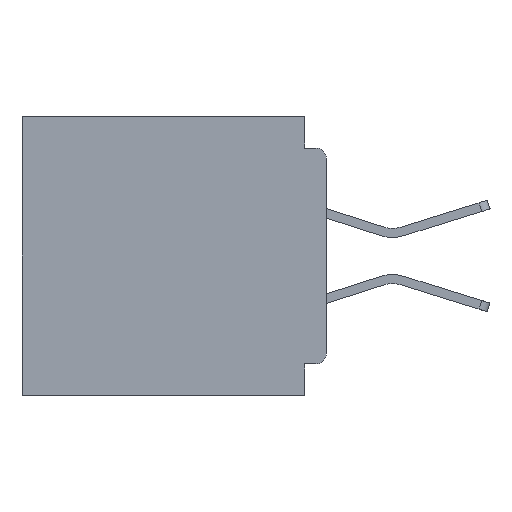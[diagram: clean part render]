
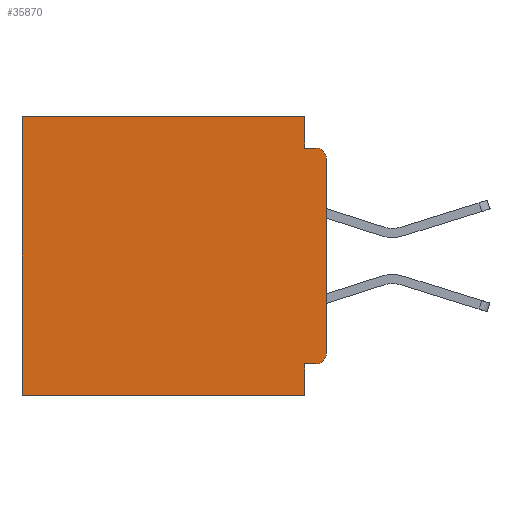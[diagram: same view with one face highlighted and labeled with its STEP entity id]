
A CAD part, left-side view. The second image highlights one B-rep face of the part: STEP entity #35870.
In plain terms, the highlighted planar face has unit normal (-1, 0, 0).
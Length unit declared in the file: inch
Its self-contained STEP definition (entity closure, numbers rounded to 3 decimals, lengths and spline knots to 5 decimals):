
#94 = VECTOR ( 'NONE', #45128, 39.37008 ) ;
#1416 = EDGE_LOOP ( 'NONE', ( #1685, #44539, #15303, #8636, #15761, #9876, #17056, #30043, #35942, #30133 ) ) ;
#1685 = ORIENTED_EDGE ( 'NONE', *, *, #7326, .F. ) ;
#1917 = VECTOR ( 'NONE', #26024, 39.37008 ) ;
#3438 = CARTESIAN_POINT ( 'NONE',  ( 0.3, 0.031, 0. ) ) ;
#3607 = PLANE ( 'NONE',  #48249 ) ;
#3907 = CARTESIAN_POINT ( 'NONE',  ( 0.3, 0.015, -0.355 ) ) ;
#5594 = CARTESIAN_POINT ( 'NONE',  ( 0.3, 0.015, -0.34 ) ) ;
#5842 = EDGE_CURVE ( 'NONE', #13653, #39688, #12678, .T. ) ;
#6872 = VECTOR ( 'NONE', #38490, 39.37008 ) ;
#7013 = VECTOR ( 'NONE', #7483, 39.37008 ) ;
#7326 = EDGE_CURVE ( 'NONE', #25076, #31655, #46342, .T. ) ;
#7483 = DIRECTION ( 'NONE',  ( 0., 0., -1. ) ) ;
#8036 = CARTESIAN_POINT ( 'NONE',  ( 0.3, 0.015, -0.06 ) ) ;
#8179 = VERTEX_POINT ( 'NONE', #11598 ) ;
#8214 = DIRECTION ( 'NONE',  ( 0., 1., 0. ) ) ;
#8307 = VERTEX_POINT ( 'NONE', #8316 ) ;
#8316 = CARTESIAN_POINT ( 'NONE',  ( 0.3, 0.437, 0. ) ) ;
#8636 = ORIENTED_EDGE ( 'NONE', *, *, #40728, .F. ) ;
#9385 = DIRECTION ( 'NONE',  ( 0., 0., -1. ) ) ;
#9876 = ORIENTED_EDGE ( 'NONE', *, *, #24919, .T. ) ;
#11168 = CARTESIAN_POINT ( 'NONE',  ( 0.3, 0., -0.4 ) ) ;
#11598 = CARTESIAN_POINT ( 'NONE',  ( 0.3, 0.031, 0. ) ) ;
#11802 = DIRECTION ( 'NONE',  ( 0., 0., -1. ) ) ;
#11887 = CARTESIAN_POINT ( 'NONE',  ( 0.3, 0.031, -0.045 ) ) ;
#11956 = EDGE_CURVE ( 'NONE', #8179, #8307, #38477, .T. ) ;
#12291 = CARTESIAN_POINT ( 'NONE',  ( 0.3, 0., -0.34 ) ) ;
#12678 = LINE ( 'NONE', #23253, #40346 ) ;
#12745 = CARTESIAN_POINT ( 'NONE',  ( 0.3, 0.031, -0.355 ) ) ;
#12749 = CIRCLE ( 'NONE', #33148, 0.015 ) ;
#13653 = VERTEX_POINT ( 'NONE', #46855 ) ;
#14889 = FACE_OUTER_BOUND ( 'NONE', #1416, .T. ) ;
#14976 = DIRECTION ( 'NONE',  ( 0., 0., -1. ) ) ;
#15303 = ORIENTED_EDGE ( 'NONE', *, *, #26352, .F. ) ;
#15761 = ORIENTED_EDGE ( 'NONE', *, *, #11956, .T. ) ;
#15949 = CARTESIAN_POINT ( 'NONE',  ( 0.3, 0.437, -0.4 ) ) ;
#16083 = EDGE_CURVE ( 'NONE', #47997, #20448, #31326, .T. ) ;
#16280 = AXIS2_PLACEMENT_3D ( 'NONE', #8036, #34402, #11802 ) ;
#17056 = ORIENTED_EDGE ( 'NONE', *, *, #5842, .F. ) ;
#17373 = CARTESIAN_POINT ( 'NONE',  ( 0.3, 0.015, -0.045 ) ) ;
#20448 = VERTEX_POINT ( 'NONE', #12745 ) ;
#20821 = LINE ( 'NONE', #3438, #1917 ) ;
#23253 = CARTESIAN_POINT ( 'NONE',  ( 0.3, 0., -0.4 ) ) ;
#23622 = EDGE_CURVE ( 'NONE', #20448, #13653, #44536, .T. ) ;
#24919 = EDGE_CURVE ( 'NONE', #8307, #39688, #38105, .T. ) ;
#25076 = VERTEX_POINT ( 'NONE', #31763 ) ;
#26024 = DIRECTION ( 'NONE',  ( 0., 0., -1. ) ) ;
#26352 = EDGE_CURVE ( 'NONE', #46736, #26911, #30128, .T. ) ;
#26911 = VERTEX_POINT ( 'NONE', #17373 ) ;
#28856 = DIRECTION ( 'NONE',  ( 0., 0., -1. ) ) ;
#29393 = EDGE_CURVE ( 'NONE', #47997, #31655, #12749, .T. ) ;
#29673 = VECTOR ( 'NONE', #47783, 39.37008 ) ;
#30043 = ORIENTED_EDGE ( 'NONE', *, *, #23622, .F. ) ;
#30069 = CARTESIAN_POINT ( 'NONE',  ( 0.3, 0.031, -0.4 ) ) ;
#30128 = LINE ( 'NONE', #36642, #40066 ) ;
#30133 = ORIENTED_EDGE ( 'NONE', *, *, #29393, .T. ) ;
#31326 = LINE ( 'NONE', #37757, #94 ) ;
#31655 = VERTEX_POINT ( 'NONE', #12291 ) ;
#31763 = CARTESIAN_POINT ( 'NONE',  ( 0.3, 0., -0.06 ) ) ;
#31967 = DIRECTION ( 'NONE',  ( -1., 0., 0. ) ) ;
#33054 = CARTESIAN_POINT ( 'NONE',  ( 0.3, 0., 0. ) ) ;
#33069 = CARTESIAN_POINT ( 'NONE',  ( 0.3, 0.437, -0.4 ) ) ;
#33148 = AXIS2_PLACEMENT_3D ( 'NONE', #5594, #31967, #9385 ) ;
#33974 = EDGE_CURVE ( 'NONE', #25076, #26911, #40294, .T. ) ;
#34402 = DIRECTION ( 'NONE',  ( -1., 0., 0. ) ) ;
#35870 = ADVANCED_FACE ( 'NONE', ( #14889 ), #3607, .F. ) ;
#35942 = ORIENTED_EDGE ( 'NONE', *, *, #16083, .F. ) ;
#36261 = CARTESIAN_POINT ( 'NONE',  ( 0.3, 0., -0.4 ) ) ;
#36537 = VECTOR ( 'NONE', #28856, 39.37008 ) ;
#36642 = CARTESIAN_POINT ( 'NONE',  ( 0.3, 0., -0.045 ) ) ;
#36806 = DIRECTION ( 'NONE',  ( 0., -1., 0. ) ) ;
#37538 = DIRECTION ( 'NONE',  ( 1., 0., 0. ) ) ;
#37757 = CARTESIAN_POINT ( 'NONE',  ( 0.3, 0., -0.355 ) ) ;
#38105 = LINE ( 'NONE', #15949, #6872 ) ;
#38477 = LINE ( 'NONE', #33054, #29673 ) ;
#38490 = DIRECTION ( 'NONE',  ( 0., 0., -1. ) ) ;
#39688 = VERTEX_POINT ( 'NONE', #33069 ) ;
#40066 = VECTOR ( 'NONE', #36806, 39.37008 ) ;
#40294 = CIRCLE ( 'NONE', #16280, 0.015 ) ;
#40346 = VECTOR ( 'NONE', #8214, 39.37008 ) ;
#40728 = EDGE_CURVE ( 'NONE', #8179, #46736, #20821, .T. ) ;
#44536 = LINE ( 'NONE', #30069, #7013 ) ;
#44539 = ORIENTED_EDGE ( 'NONE', *, *, #33974, .T. ) ;
#45128 = DIRECTION ( 'NONE',  ( 0., 1., 0. ) ) ;
#46342 = LINE ( 'NONE', #36261, #36537 ) ;
#46736 = VERTEX_POINT ( 'NONE', #11887 ) ;
#46855 = CARTESIAN_POINT ( 'NONE',  ( 0.3, 0.031, -0.4 ) ) ;
#47783 = DIRECTION ( 'NONE',  ( 0., 1., 0. ) ) ;
#47997 = VERTEX_POINT ( 'NONE', #3907 ) ;
#48249 = AXIS2_PLACEMENT_3D ( 'NONE', #11168, #37538, #14976 ) ;
